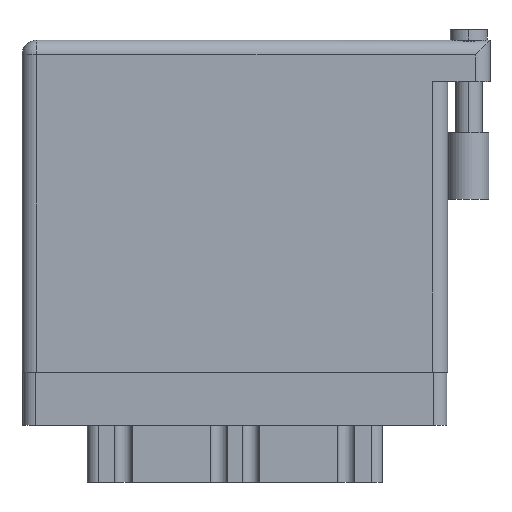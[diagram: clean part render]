
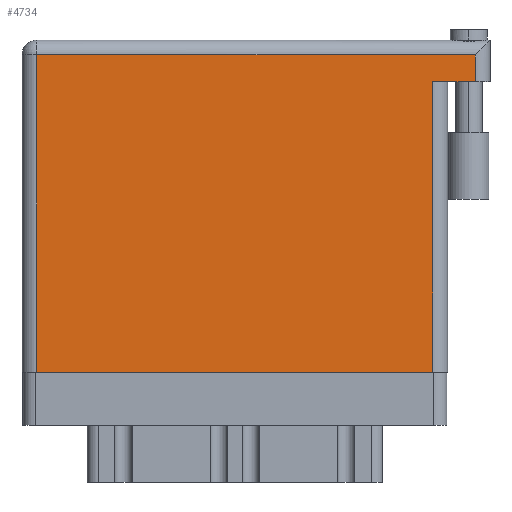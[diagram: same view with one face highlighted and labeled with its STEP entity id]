
A CAD part, front view. The second image highlights one B-rep face of the part: STEP entity #4734.
In plain terms, the highlighted face is planar.
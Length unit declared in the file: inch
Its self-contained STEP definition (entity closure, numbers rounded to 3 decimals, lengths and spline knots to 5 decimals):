
#280 = VECTOR ( 'NONE', #33693, 39.37008 ) ;
#589 = VECTOR ( 'NONE', #5341, 39.37008 ) ;
#981 = CARTESIAN_POINT ( 'NONE',  ( 1.938, 1.369, 0. ) ) ;
#2686 = ORIENTED_EDGE ( 'NONE', *, *, #22673, .T. ) ;
#2904 = VERTEX_POINT ( 'NONE', #33895 ) ;
#4734 = ADVANCED_FACE ( 'NONE', ( #33425 ), #10135, .F. ) ;
#4829 = VERTEX_POINT ( 'NONE', #5241 ) ;
#5241 = CARTESIAN_POINT ( 'NONE',  ( 1.938, 1.369, 0. ) ) ;
#5341 = DIRECTION ( 'NONE',  ( 1., 0., 0. ) ) ;
#7205 = CARTESIAN_POINT ( 'NONE',  ( 0., 1.566, 0. ) ) ;
#8284 = CARTESIAN_POINT ( 'NONE',  ( 0., 0., 0. ) ) ;
#8461 = ORIENTED_EDGE ( 'NONE', *, *, #10734, .F. ) ;
#8793 = CARTESIAN_POINT ( 'NONE',  ( 2.208, 1.369, 0. ) ) ;
#9880 = EDGE_CURVE ( 'NONE', #19503, #2904, #34894, .T. ) ;
#10135 = PLANE ( 'NONE',  #31585 ) ;
#10734 = EDGE_CURVE ( 'NONE', #14525, #4829, #20244, .T. ) ;
#12007 = CARTESIAN_POINT ( 'NONE',  ( 0.07, 1.496, 0. ) ) ;
#13534 = EDGE_CURVE ( 'NONE', #14525, #27977, #32043, .T. ) ;
#14394 = VECTOR ( 'NONE', #24109, 39.37008 ) ;
#14525 = VERTEX_POINT ( 'NONE', #23974 ) ;
#14597 = CARTESIAN_POINT ( 'NONE',  ( 0., 1.496, 0. ) ) ;
#14814 = CARTESIAN_POINT ( 'NONE',  ( 2.138, 1.496, 0. ) ) ;
#16642 = ORIENTED_EDGE ( 'NONE', *, *, #9880, .T. ) ;
#19503 = VERTEX_POINT ( 'NONE', #32300 ) ;
#19833 = VERTEX_POINT ( 'NONE', #12007 ) ;
#20244 = LINE ( 'NONE', #8793, #34441 ) ;
#20790 = DIRECTION ( 'NONE',  ( -1., 0., 0. ) ) ;
#21770 = ORIENTED_EDGE ( 'NONE', *, *, #24294, .T. ) ;
#22023 = DIRECTION ( 'NONE',  ( 0., -1., 0. ) ) ;
#22164 = DIRECTION ( 'NONE',  ( 0., 0., -1. ) ) ;
#22673 = EDGE_CURVE ( 'NONE', #2904, #4829, #30115, .T. ) ;
#23974 = CARTESIAN_POINT ( 'NONE',  ( 2.138, 1.369, 0. ) ) ;
#24109 = DIRECTION ( 'NONE',  ( 0., 1., 0. ) ) ;
#24294 = EDGE_CURVE ( 'NONE', #27977, #19833, #29334, .T. ) ;
#27977 = VERTEX_POINT ( 'NONE', #14814 ) ;
#29143 = CARTESIAN_POINT ( 'NONE',  ( 2.138, 1.566, 0. ) ) ;
#29334 = LINE ( 'NONE', #14597, #31741 ) ;
#29556 = DIRECTION ( 'NONE',  ( -1., 0., 0. ) ) ;
#30115 = LINE ( 'NONE', #981, #14394 ) ;
#30341 = VECTOR ( 'NONE', #22023, 39.37008 ) ;
#30751 = CARTESIAN_POINT ( 'NONE',  ( 0.07, 0., 0. ) ) ;
#31082 = DIRECTION ( 'NONE',  ( -1., 0., 0. ) ) ;
#31585 = AXIS2_PLACEMENT_3D ( 'NONE', #7205, #22164, #31082 ) ;
#31741 = VECTOR ( 'NONE', #20790, 39.37008 ) ;
#32043 = LINE ( 'NONE', #29143, #280 ) ;
#32300 = CARTESIAN_POINT ( 'NONE',  ( 0.07, 0., 0. ) ) ;
#32304 = ORIENTED_EDGE ( 'NONE', *, *, #13534, .T. ) ;
#33425 = FACE_OUTER_BOUND ( 'NONE', #34649, .T. ) ;
#33693 = DIRECTION ( 'NONE',  ( 0., 1., 0. ) ) ;
#33895 = CARTESIAN_POINT ( 'NONE',  ( 1.938, 0., 0. ) ) ;
#34441 = VECTOR ( 'NONE', #29556, 39.37008 ) ;
#34649 = EDGE_LOOP ( 'NONE', ( #16642, #2686, #8461, #32304, #21770, #37804 ) ) ;
#34894 = LINE ( 'NONE', #8284, #589 ) ;
#36147 = EDGE_CURVE ( 'NONE', #19833, #19503, #37155, .T. ) ;
#37155 = LINE ( 'NONE', #30751, #30341 ) ;
#37804 = ORIENTED_EDGE ( 'NONE', *, *, #36147, .T. ) ;
